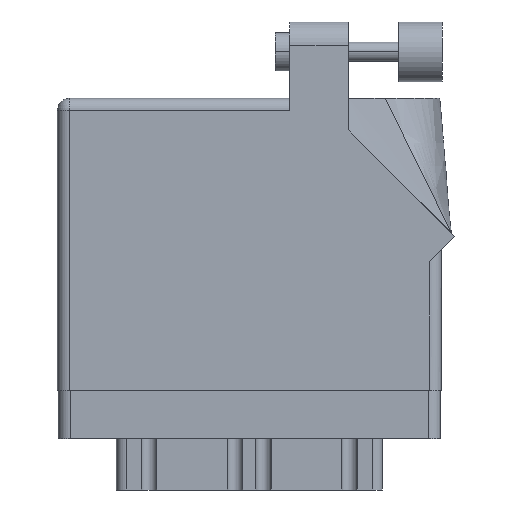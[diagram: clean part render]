
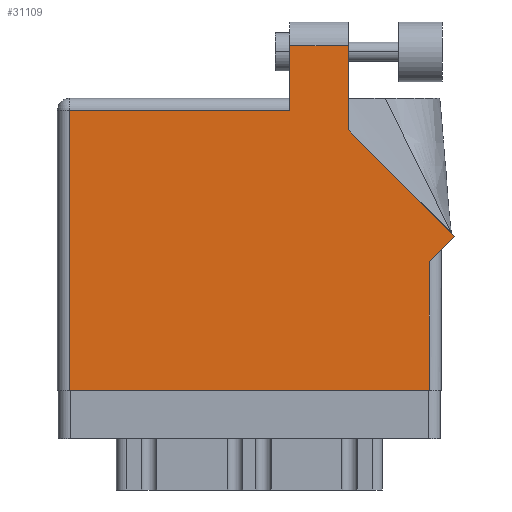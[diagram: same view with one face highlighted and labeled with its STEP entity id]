
A CAD part, front view. The second image highlights one B-rep face of the part: STEP entity #31109.
In plain terms, the highlighted face is planar.
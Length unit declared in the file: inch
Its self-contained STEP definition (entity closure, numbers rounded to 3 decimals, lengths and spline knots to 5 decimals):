
#258 = VERTEX_POINT ( 'NONE', #12688 ) ;
#475 = LINE ( 'NONE', #32532, #6476 ) ;
#2994 = VECTOR ( 'NONE', #33992, 39.37008 ) ;
#3094 = CARTESIAN_POINT ( 'NONE',  ( 0., 0., 0. ) ) ;
#3100 = VERTEX_POINT ( 'NONE', #9205 ) ;
#3456 = CARTESIAN_POINT ( 'NONE',  ( 1.217, 1.805, 0. ) ) ;
#3953 = EDGE_CURVE ( 'NONE', #22627, #18182, #7747, .T. ) ;
#4132 = ORIENTED_EDGE ( 'NONE', *, *, #10463, .T. ) ;
#5205 = VECTOR ( 'NONE', #7081, 39.37008 ) ;
#5417 = PLANE ( 'NONE',  #30473 ) ;
#6476 = VECTOR ( 'NONE', #8546, 39.37008 ) ;
#7081 = DIRECTION ( 'NONE',  ( 0.707, 0.707, 0. ) ) ;
#7309 = VERTEX_POINT ( 'NONE', #11443 ) ;
#7428 = LINE ( 'NONE', #31077, #5205 ) ;
#7747 = LINE ( 'NONE', #3094, #25539 ) ;
#7847 = VECTOR ( 'NONE', #18567, 39.37008 ) ;
#7941 = CARTESIAN_POINT ( 'NONE',  ( 1.948, 0.737, 0. ) ) ;
#7954 = EDGE_CURVE ( 'NONE', #7309, #258, #12597, .T. ) ;
#8546 = DIRECTION ( 'NONE',  ( -1., 0., 0. ) ) ;
#9205 = CARTESIAN_POINT ( 'NONE',  ( 1.948, 0.675, 0. ) ) ;
#10463 = EDGE_CURVE ( 'NONE', #29099, #26175, #475, .T. ) ;
#10565 = VECTOR ( 'NONE', #23394, 39.37008 ) ;
#11356 = ORIENTED_EDGE ( 'NONE', *, *, #25960, .T. ) ;
#11443 = CARTESIAN_POINT ( 'NONE',  ( 2.08071, 0.80771, 0. ) ) ;
#12597 = LINE ( 'NONE', #23284, #7847 ) ;
#12688 = CARTESIAN_POINT ( 'NONE',  ( 1.524, 1.36442, 0. ) ) ;
#14913 = EDGE_CURVE ( 'NONE', #258, #34488, #30814, .T. ) ;
#15333 = ORIENTED_EDGE ( 'NONE', *, *, #24680, .T. ) ;
#15434 = DIRECTION ( 'NONE',  ( -1., 0., 0. ) ) ;
#16143 = FACE_OUTER_BOUND ( 'NONE', #17564, .T. ) ;
#17564 = EDGE_LOOP ( 'NONE', ( #28900, #11356, #15333, #4132, #27769, #29852, #21298, #23402, #28418 ) ) ;
#17814 = CARTESIAN_POINT ( 'NONE',  ( 1.524, 1.805, 0. ) ) ;
#17992 = CARTESIAN_POINT ( 'NONE',  ( 0.062, 0., 0. ) ) ;
#18182 = VERTEX_POINT ( 'NONE', #29817 ) ;
#18454 = DIRECTION ( 'NONE',  ( 1., 0., 0. ) ) ;
#18567 = DIRECTION ( 'NONE',  ( -0.707, 0.707, 0. ) ) ;
#18591 = DIRECTION ( 'NONE',  ( 0., 0., -1. ) ) ;
#19736 = VERTEX_POINT ( 'NONE', #3456 ) ;
#20035 = CARTESIAN_POINT ( 'NONE',  ( 0.062, 1.468, 0. ) ) ;
#20141 = EDGE_CURVE ( 'NONE', #3100, #7309, #7428, .T. ) ;
#20155 = CARTESIAN_POINT ( 'NONE',  ( 1.524, 1.36442, 0. ) ) ;
#21298 = ORIENTED_EDGE ( 'NONE', *, *, #23271, .T. ) ;
#22267 = DIRECTION ( 'NONE',  ( 0., 1., 0. ) ) ;
#22627 = VERTEX_POINT ( 'NONE', #17992 ) ;
#23021 = LINE ( 'NONE', #33718, #23872 ) ;
#23024 = CARTESIAN_POINT ( 'NONE',  ( 1.217, 1.805, 0. ) ) ;
#23271 = EDGE_CURVE ( 'NONE', #18182, #3100, #26678, .T. ) ;
#23284 = CARTESIAN_POINT ( 'NONE',  ( 2.08071, 0.80771, 0. ) ) ;
#23291 = CARTESIAN_POINT ( 'NONE',  ( 0.062, 0., 0. ) ) ;
#23394 = DIRECTION ( 'NONE',  ( -1., 0., 0. ) ) ;
#23402 = ORIENTED_EDGE ( 'NONE', *, *, #20141, .T. ) ;
#23828 = LINE ( 'NONE', #23291, #2994 ) ;
#23872 = VECTOR ( 'NONE', #31425, 39.37008 ) ;
#24596 = CARTESIAN_POINT ( 'NONE',  ( 1.217, 1.468, 0. ) ) ;
#24680 = EDGE_CURVE ( 'NONE', #19736, #29099, #23021, .T. ) ;
#25539 = VECTOR ( 'NONE', #18454, 39.37008 ) ;
#25960 = EDGE_CURVE ( 'NONE', #34488, #19736, #26349, .T. ) ;
#26175 = VERTEX_POINT ( 'NONE', #20035 ) ;
#26349 = LINE ( 'NONE', #23024, #10565 ) ;
#26678 = LINE ( 'NONE', #7941, #27107 ) ;
#27107 = VECTOR ( 'NONE', #22267, 39.37008 ) ;
#27769 = ORIENTED_EDGE ( 'NONE', *, *, #28531, .T. ) ;
#28418 = ORIENTED_EDGE ( 'NONE', *, *, #7954, .T. ) ;
#28440 = VECTOR ( 'NONE', #33468, 39.37008 ) ;
#28531 = EDGE_CURVE ( 'NONE', #26175, #22627, #23828, .T. ) ;
#28900 = ORIENTED_EDGE ( 'NONE', *, *, #14913, .T. ) ;
#29099 = VERTEX_POINT ( 'NONE', #24596 ) ;
#29423 = CARTESIAN_POINT ( 'NONE',  ( 0., 1.53, 0. ) ) ;
#29817 = CARTESIAN_POINT ( 'NONE',  ( 1.948, 0., 0. ) ) ;
#29852 = ORIENTED_EDGE ( 'NONE', *, *, #3953, .T. ) ;
#30473 = AXIS2_PLACEMENT_3D ( 'NONE', #29423, #18591, #15434 ) ;
#30814 = LINE ( 'NONE', #20155, #28440 ) ;
#31077 = CARTESIAN_POINT ( 'NONE',  ( 2.01, 0.737, 0. ) ) ;
#31109 = ADVANCED_FACE ( 'NONE', ( #16143 ), #5417, .F. ) ;
#31425 = DIRECTION ( 'NONE',  ( 0., -1., 0. ) ) ;
#32532 = CARTESIAN_POINT ( 'NONE',  ( 0., 1.468, 0. ) ) ;
#33468 = DIRECTION ( 'NONE',  ( 0., 1., 0. ) ) ;
#33718 = CARTESIAN_POINT ( 'NONE',  ( 1.217, 1.53, 0. ) ) ;
#33992 = DIRECTION ( 'NONE',  ( 0., -1., 0. ) ) ;
#34488 = VERTEX_POINT ( 'NONE', #17814 ) ;
